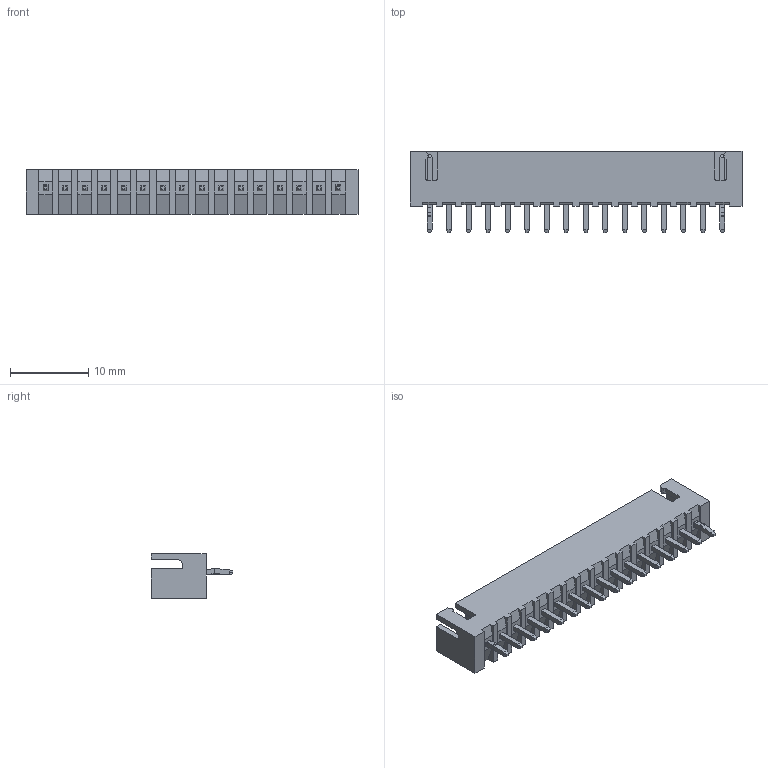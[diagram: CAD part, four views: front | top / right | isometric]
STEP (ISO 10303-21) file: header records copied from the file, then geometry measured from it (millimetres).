
FILE_DESCRIPTION (( 'STEP AP203' ), '1' );
FILE_NAME ('14K-516-411-AA1.STEP', '2024-02-23T17:04:44', ( '' ), ( '' ), 'SwSTEP 2.0', 'SolidWorks 2023', '' );
FILE_SCHEMA (( 'CONFIG_CONTROL_DESIGN' ));
Length unit declared in the file: millimetre
Products named in the file (4): 14K Series Pin_15; 14K Series Pin_11; 14K Series Pin Header Insulator_516; 14K-516-411-AA1
Assembly tree (17 placements, depth 2):
  14K-516-411-AA1
    14K Series Pin Header Insulator_516
    14K Series Pin_11  x2
    14K Series Pin_15  x14
Bounding box: 42.5 x 10.4 x 5.75 mm (x, y, z)
Volume: 781.6 mm3; surface area: 2126.2 mm2
Topology: 17 solids, 17 shells, 492 faces, 1238 edges, 780 vertices
Faces by surface type: plane 471, cylinder 21
Entity records: 8900 total; most frequent: CARTESIAN_POINT 1450, ORIENTED_EDGE 1424, DIRECTION 1290, EDGE_CURVE 712, LINE 674, VECTOR 674, VERTEX_POINT 468, AXIS2_PLACEMENT_3D 308
